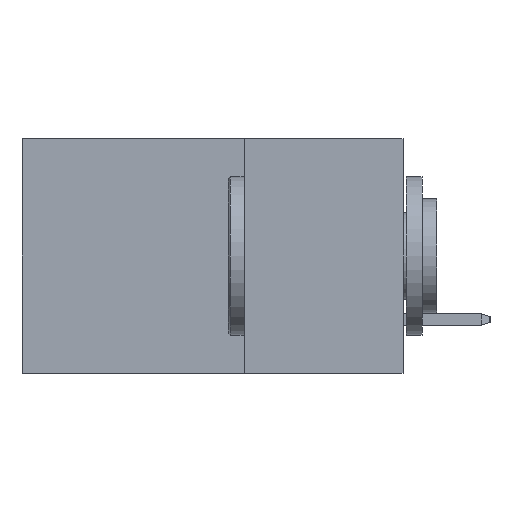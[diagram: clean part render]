
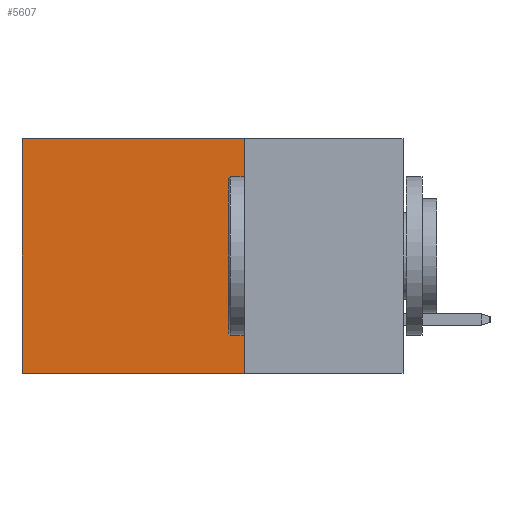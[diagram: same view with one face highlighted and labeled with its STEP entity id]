
A CAD part, left-side view. The second image highlights one B-rep face of the part: STEP entity #5607.
In plain terms, the highlighted planar face has unit normal (-1, 0, 0).
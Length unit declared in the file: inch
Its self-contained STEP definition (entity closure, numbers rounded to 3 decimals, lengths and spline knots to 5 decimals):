
#827 = VECTOR ( 'NONE', #6445, 39.37008 ) ;
#2899 = ORIENTED_EDGE ( 'NONE', *, *, #12341, .F. ) ;
#3010 = VERTEX_POINT ( 'NONE', #14532 ) ;
#3149 = CARTESIAN_POINT ( 'NONE',  ( 0.2875, 0.6, 0. ) ) ;
#3163 = EDGE_CURVE ( 'NONE', #3010, #15277, #16399, .T. ) ;
#3945 = FACE_OUTER_BOUND ( 'NONE', #14242, .T. ) ;
#4191 = ORIENTED_EDGE ( 'NONE', *, *, #9989, .T. ) ;
#5607 = ADVANCED_FACE ( 'NONE', ( #3945 ), #11823, .F. ) ;
#6224 = VECTOR ( 'NONE', #14231, 39.37008 ) ;
#6445 = DIRECTION ( 'NONE',  ( 0., 0., -1. ) ) ;
#7699 = AXIS2_PLACEMENT_3D ( 'NONE', #15998, #9533, #15920 ) ;
#7830 = ORIENTED_EDGE ( 'NONE', *, *, #15463, .T. ) ;
#7860 = CARTESIAN_POINT ( 'NONE',  ( 0.2875, 0.25, 0. ) ) ;
#8386 = VERTEX_POINT ( 'NONE', #3149 ) ;
#8579 = CARTESIAN_POINT ( 'NONE',  ( 0.2875, 0.25, -0.37 ) ) ;
#9533 = DIRECTION ( 'NONE',  ( 1., 0., 0. ) ) ;
#9989 = EDGE_CURVE ( 'NONE', #15964, #8386, #11612, .T. ) ;
#10295 = CARTESIAN_POINT ( 'NONE',  ( 0.2875, 0.25, 0. ) ) ;
#11612 = LINE ( 'NONE', #11701, #14371 ) ;
#11643 = LINE ( 'NONE', #11894, #827 ) ;
#11701 = CARTESIAN_POINT ( 'NONE',  ( 0.2875, 0.25, 0. ) ) ;
#11823 = PLANE ( 'NONE',  #7699 ) ;
#11894 = CARTESIAN_POINT ( 'NONE',  ( 0.2875, 0.6, 0. ) ) ;
#12341 = EDGE_CURVE ( 'NONE', #15964, #3010, #15411, .T. ) ;
#12522 = VECTOR ( 'NONE', #13762, 39.37008 ) ;
#13762 = DIRECTION ( 'NONE',  ( 0., 1., 0. ) ) ;
#14231 = DIRECTION ( 'NONE',  ( 0., 0., -1. ) ) ;
#14242 = EDGE_LOOP ( 'NONE', ( #7830, #14320, #2899, #4191 ) ) ;
#14320 = ORIENTED_EDGE ( 'NONE', *, *, #3163, .F. ) ;
#14371 = VECTOR ( 'NONE', #16821, 39.37008 ) ;
#14532 = CARTESIAN_POINT ( 'NONE',  ( 0.2875, 0.25, -0.37 ) ) ;
#15277 = VERTEX_POINT ( 'NONE', #16012 ) ;
#15411 = LINE ( 'NONE', #10295, #6224 ) ;
#15463 = EDGE_CURVE ( 'NONE', #8386, #15277, #11643, .T. ) ;
#15920 = DIRECTION ( 'NONE',  ( 0., 0., -1. ) ) ;
#15964 = VERTEX_POINT ( 'NONE', #7860 ) ;
#15998 = CARTESIAN_POINT ( 'NONE',  ( 0.2875, 0.25, 0. ) ) ;
#16012 = CARTESIAN_POINT ( 'NONE',  ( 0.2875, 0.6, -0.37 ) ) ;
#16399 = LINE ( 'NONE', #8579, #12522 ) ;
#16821 = DIRECTION ( 'NONE',  ( 0., 1., 0. ) ) ;
